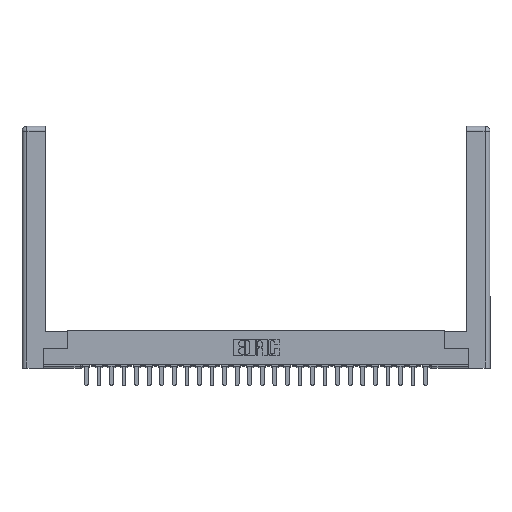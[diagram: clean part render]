
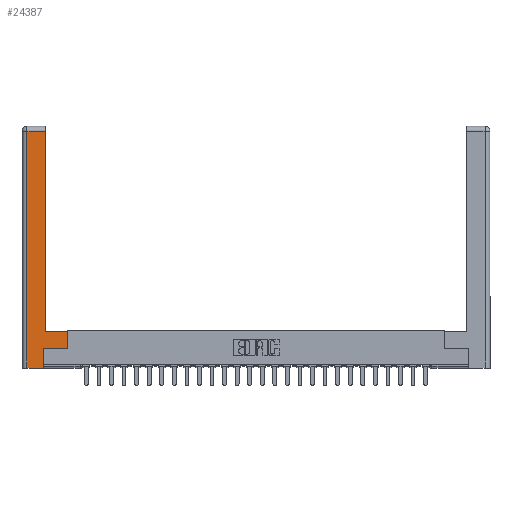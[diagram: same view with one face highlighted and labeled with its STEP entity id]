
A CAD part, top view. The second image highlights one B-rep face of the part: STEP entity #24387.
In plain terms, the highlighted planar face has unit normal (0, 0, 1).
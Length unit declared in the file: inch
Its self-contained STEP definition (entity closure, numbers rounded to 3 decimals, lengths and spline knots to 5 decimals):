
#182 = LINE ( 'NONE', #17311, #16346 ) ;
#532 = LINE ( 'NONE', #8110, #23728 ) ;
#569 = ORIENTED_EDGE ( 'NONE', *, *, #26455, .T. ) ;
#1726 = VECTOR ( 'NONE', #17183, 39.37008 ) ;
#2121 = CARTESIAN_POINT ( 'NONE',  ( 0., 0., 0. ) ) ;
#2942 = EDGE_LOOP ( 'NONE', ( #22420, #24917, #13473, #19707, #569, #27548, #8571, #3181 ) ) ;
#3181 = ORIENTED_EDGE ( 'NONE', *, *, #3940, .T. ) ;
#3403 = DIRECTION ( 'NONE',  ( 1., 0., 0. ) ) ;
#3940 = EDGE_CURVE ( 'NONE', #8844, #21086, #182, .T. ) ;
#3984 = LINE ( 'NONE', #21550, #15622 ) ;
#5411 = LINE ( 'NONE', #10084, #23311 ) ;
#5636 = VECTOR ( 'NONE', #3403, 39.37008 ) ;
#6261 = VECTOR ( 'NONE', #8328, 39.37008 ) ;
#6361 = CARTESIAN_POINT ( 'NONE',  ( 0.565, 0.245, 0. ) ) ;
#6506 = AXIS2_PLACEMENT_3D ( 'NONE', #2121, #11275, #15708 ) ;
#7705 = LINE ( 'NONE', #12646, #22132 ) ;
#7971 = CARTESIAN_POINT ( 'NONE',  ( 0.265, 0., 0. ) ) ;
#8110 = CARTESIAN_POINT ( 'NONE',  ( 0.565, 0.245, 0. ) ) ;
#8207 = DIRECTION ( 'NONE',  ( 0., 1., 0. ) ) ;
#8323 = CARTESIAN_POINT ( 'NONE',  ( 0.0615, 2.94, 0. ) ) ;
#8328 = DIRECTION ( 'NONE',  ( 0., -1., 0. ) ) ;
#8520 = VERTEX_POINT ( 'NONE', #27353 ) ;
#8571 = ORIENTED_EDGE ( 'NONE', *, *, #17338, .T. ) ;
#8844 = VERTEX_POINT ( 'NONE', #14482 ) ;
#8937 = VERTEX_POINT ( 'NONE', #7971 ) ;
#10084 = CARTESIAN_POINT ( 'NONE',  ( 0.295, 3., 0. ) ) ;
#11052 = CARTESIAN_POINT ( 'NONE',  ( 0.265, 0.245, 0. ) ) ;
#11275 = DIRECTION ( 'NONE',  ( 0., 0., -1. ) ) ;
#11573 = LINE ( 'NONE', #16873, #5636 ) ;
#12104 = VERTEX_POINT ( 'NONE', #6361 ) ;
#12116 = VERTEX_POINT ( 'NONE', #26627 ) ;
#12646 = CARTESIAN_POINT ( 'NONE',  ( 0.565, 0.45, 0. ) ) ;
#13473 = ORIENTED_EDGE ( 'NONE', *, *, #28561, .T. ) ;
#13586 = VERTEX_POINT ( 'NONE', #11052 ) ;
#14482 = CARTESIAN_POINT ( 'NONE',  ( 0.565, 0.45, 0. ) ) ;
#14731 = LINE ( 'NONE', #8323, #1726 ) ;
#15622 = VECTOR ( 'NONE', #8207, 39.37008 ) ;
#15708 = DIRECTION ( 'NONE',  ( -1., 0., 0. ) ) ;
#16346 = VECTOR ( 'NONE', #28554, 39.37008 ) ;
#16873 = CARTESIAN_POINT ( 'NONE',  ( 0.265, 0., 0. ) ) ;
#17075 = CARTESIAN_POINT ( 'NONE',  ( 0.0615, 0., 0. ) ) ;
#17183 = DIRECTION ( 'NONE',  ( -1., 0., 0. ) ) ;
#17311 = CARTESIAN_POINT ( 'NONE',  ( 0.295, 0.45, 0. ) ) ;
#17338 = EDGE_CURVE ( 'NONE', #12104, #8844, #7705, .T. ) ;
#18877 = FACE_OUTER_BOUND ( 'NONE', #2942, .T. ) ;
#19059 = DIRECTION ( 'NONE',  ( 0., 1., 0. ) ) ;
#19707 = ORIENTED_EDGE ( 'NONE', *, *, #22690, .T. ) ;
#19972 = DIRECTION ( 'NONE',  ( 1., 0., 0. ) ) ;
#20617 = LINE ( 'NONE', #17075, #6261 ) ;
#21086 = VERTEX_POINT ( 'NONE', #25055 ) ;
#21458 = DIRECTION ( 'NONE',  ( 0., 1., 0. ) ) ;
#21550 = CARTESIAN_POINT ( 'NONE',  ( 0.265, 0.245, 0. ) ) ;
#22132 = VECTOR ( 'NONE', #19059, 39.37008 ) ;
#22420 = ORIENTED_EDGE ( 'NONE', *, *, #26491, .T. ) ;
#22690 = EDGE_CURVE ( 'NONE', #12116, #8937, #11573, .T. ) ;
#22807 = EDGE_CURVE ( 'NONE', #24332, #8520, #14731, .T. ) ;
#23311 = VECTOR ( 'NONE', #21458, 39.37008 ) ;
#23728 = VECTOR ( 'NONE', #19972, 39.37008 ) ;
#24332 = VERTEX_POINT ( 'NONE', #24787 ) ;
#24387 = ADVANCED_FACE ( 'NONE', ( #18877 ), #24696, .F. ) ;
#24696 = PLANE ( 'NONE',  #6506 ) ;
#24787 = CARTESIAN_POINT ( 'NONE',  ( 0.295, 2.94, 0. ) ) ;
#24854 = EDGE_CURVE ( 'NONE', #13586, #12104, #532, .T. ) ;
#24917 = ORIENTED_EDGE ( 'NONE', *, *, #22807, .T. ) ;
#25055 = CARTESIAN_POINT ( 'NONE',  ( 0.295, 0.45, 0. ) ) ;
#26455 = EDGE_CURVE ( 'NONE', #8937, #13586, #3984, .T. ) ;
#26491 = EDGE_CURVE ( 'NONE', #21086, #24332, #5411, .T. ) ;
#26627 = CARTESIAN_POINT ( 'NONE',  ( 0.0615, 0., 0. ) ) ;
#27353 = CARTESIAN_POINT ( 'NONE',  ( 0.0615, 2.94, 0. ) ) ;
#27548 = ORIENTED_EDGE ( 'NONE', *, *, #24854, .T. ) ;
#28554 = DIRECTION ( 'NONE',  ( -1., 0., 0. ) ) ;
#28561 = EDGE_CURVE ( 'NONE', #8520, #12116, #20617, .T. ) ;
